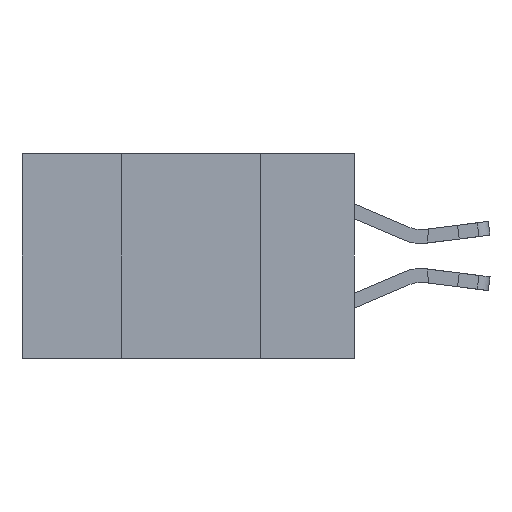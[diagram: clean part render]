
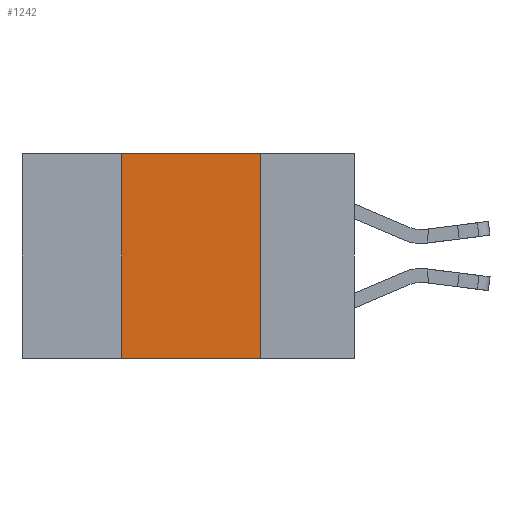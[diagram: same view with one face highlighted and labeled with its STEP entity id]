
A CAD part, left-side view. The second image highlights one B-rep face of the part: STEP entity #1242.
In plain terms, the highlighted planar face has unit normal (-1, 0, 0).
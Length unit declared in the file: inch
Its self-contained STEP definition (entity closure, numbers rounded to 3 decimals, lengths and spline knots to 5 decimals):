
#206 = CARTESIAN_POINT ( 'NONE',  ( 0., 0.42, 0. ) ) ;
#221 = VERTEX_POINT ( 'NONE', #9004 ) ;
#761 = EDGE_CURVE ( 'NONE', #6649, #5966, #5397, .T. ) ;
#871 = CARTESIAN_POINT ( 'NONE',  ( 0., 0.42, -0.37 ) ) ;
#1242 = ADVANCED_FACE ( 'NONE', ( #6960 ), #7605, .F. ) ;
#1246 = EDGE_CURVE ( 'NONE', #6649, #5716, #8591, .T. ) ;
#1757 = ORIENTED_EDGE ( 'NONE', *, *, #1246, .F. ) ;
#2228 = CARTESIAN_POINT ( 'NONE',  ( 0., 0.42, -0.37 ) ) ;
#4236 = VECTOR ( 'NONE', #6952, 39.37008 ) ;
#4443 = CARTESIAN_POINT ( 'NONE',  ( 0., 0.6, 0. ) ) ;
#4762 = LINE ( 'NONE', #4443, #4236 ) ;
#5397 = LINE ( 'NONE', #7197, #9536 ) ;
#5716 = VERTEX_POINT ( 'NONE', #206 ) ;
#5749 = CARTESIAN_POINT ( 'NONE',  ( 0., 0.17, -0.37 ) ) ;
#5886 = ORIENTED_EDGE ( 'NONE', *, *, #6736, .F. ) ;
#5966 = VERTEX_POINT ( 'NONE', #9932 ) ;
#6155 = AXIS2_PLACEMENT_3D ( 'NONE', #9354, #7100, #7128 ) ;
#6247 = EDGE_CURVE ( 'NONE', #5716, #221, #4762, .T. ) ;
#6601 = DIRECTION ( 'NONE',  ( 0., 0., -1. ) ) ;
#6649 = VERTEX_POINT ( 'NONE', #2228 ) ;
#6736 = EDGE_CURVE ( 'NONE', #221, #5966, #6968, .T. ) ;
#6840 = ORIENTED_EDGE ( 'NONE', *, *, #6247, .F. ) ;
#6952 = DIRECTION ( 'NONE',  ( 0., -1., 0. ) ) ;
#6960 = FACE_OUTER_BOUND ( 'NONE', #9333, .T. ) ;
#6968 = LINE ( 'NONE', #5749, #8870 ) ;
#7100 = DIRECTION ( 'NONE',  ( 1., 0., 0. ) ) ;
#7128 = DIRECTION ( 'NONE',  ( 0., 0., -1. ) ) ;
#7197 = CARTESIAN_POINT ( 'NONE',  ( 0., 0.6, -0.37 ) ) ;
#7605 = PLANE ( 'NONE',  #6155 ) ;
#7617 = DIRECTION ( 'NONE',  ( 0., 0., 1. ) ) ;
#8591 = LINE ( 'NONE', #871, #10723 ) ;
#8870 = VECTOR ( 'NONE', #6601, 39.37008 ) ;
#9004 = CARTESIAN_POINT ( 'NONE',  ( 0., 0.17, 0. ) ) ;
#9333 = EDGE_LOOP ( 'NONE', ( #5886, #6840, #1757, #9418 ) ) ;
#9354 = CARTESIAN_POINT ( 'NONE',  ( 0., 0.6, 0. ) ) ;
#9418 = ORIENTED_EDGE ( 'NONE', *, *, #761, .T. ) ;
#9536 = VECTOR ( 'NONE', #9826, 39.37008 ) ;
#9826 = DIRECTION ( 'NONE',  ( 0., -1., 0. ) ) ;
#9932 = CARTESIAN_POINT ( 'NONE',  ( 0., 0.17, -0.37 ) ) ;
#10723 = VECTOR ( 'NONE', #7617, 39.37008 ) ;
